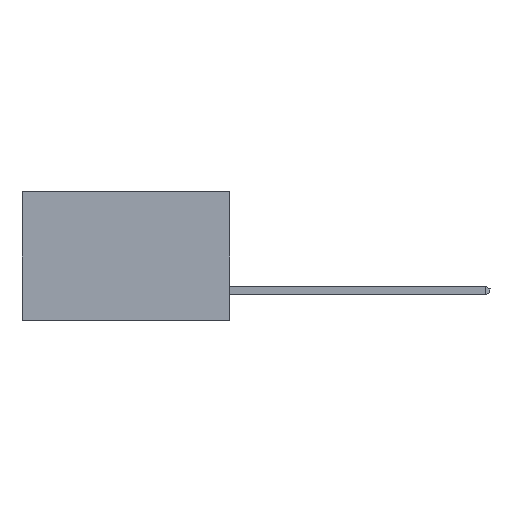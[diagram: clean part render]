
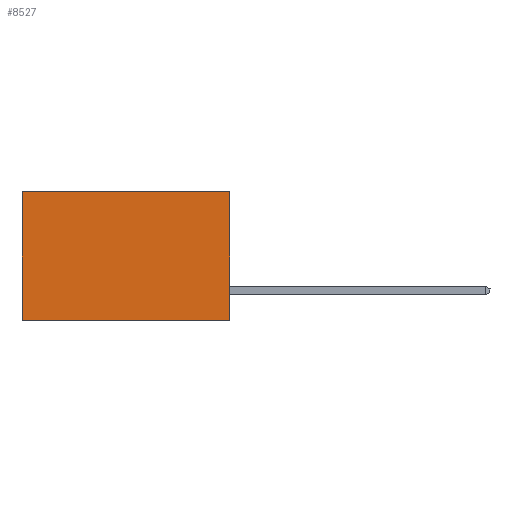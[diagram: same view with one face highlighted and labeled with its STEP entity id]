
A CAD part, left-side view. The second image highlights one B-rep face of the part: STEP entity #8527.
In plain terms, the highlighted planar face has unit normal (-1, 0, 0).
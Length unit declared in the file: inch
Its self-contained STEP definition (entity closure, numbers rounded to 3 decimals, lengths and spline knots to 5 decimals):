
#136 = LINE ( 'NONE', #9675, #4536 ) ;
#439 = VECTOR ( 'NONE', #9544, 39.37008 ) ;
#2019 = VERTEX_POINT ( 'NONE', #7161 ) ;
#2133 = FACE_OUTER_BOUND ( 'NONE', #12678, .T. ) ;
#2327 = ORIENTED_EDGE ( 'NONE', *, *, #19947, .F. ) ;
#3469 = VECTOR ( 'NONE', #21850, 39.37008 ) ;
#3531 = DIRECTION ( 'NONE',  ( 0., 1., 0. ) ) ;
#4450 = DIRECTION ( 'NONE',  ( 0., 0., -1. ) ) ;
#4536 = VECTOR ( 'NONE', #9619, 39.37008 ) ;
#5039 = DIRECTION ( 'NONE',  ( 1., 0., 0. ) ) ;
#5213 = CARTESIAN_POINT ( 'NONE',  ( 0.2615, 0.6, 0. ) ) ;
#5309 = CARTESIAN_POINT ( 'NONE',  ( 0.2615, 0., -0.37 ) ) ;
#5586 = CARTESIAN_POINT ( 'NONE',  ( 0.2615, 0., 0. ) ) ;
#6107 = PLANE ( 'NONE',  #15136 ) ;
#6421 = EDGE_CURVE ( 'NONE', #7771, #11549, #136, .T. ) ;
#7161 = CARTESIAN_POINT ( 'NONE',  ( 0.2615, 0., -0.37 ) ) ;
#7721 = CARTESIAN_POINT ( 'NONE',  ( 0.2615, 0., -0.37 ) ) ;
#7771 = VERTEX_POINT ( 'NONE', #5213 ) ;
#8527 = ADVANCED_FACE ( 'NONE', ( #2133 ), #6107, .F. ) ;
#9544 = DIRECTION ( 'NONE',  ( 0., 1., 0. ) ) ;
#9549 = ORIENTED_EDGE ( 'NONE', *, *, #15343, .T. ) ;
#9619 = DIRECTION ( 'NONE',  ( 0., 0., -1. ) ) ;
#9675 = CARTESIAN_POINT ( 'NONE',  ( 0.2615, 0.6, -0.37 ) ) ;
#10107 = VERTEX_POINT ( 'NONE', #5586 ) ;
#10223 = LINE ( 'NONE', #7721, #439 ) ;
#11531 = CARTESIAN_POINT ( 'NONE',  ( 0.2615, 0., -0.37 ) ) ;
#11549 = VERTEX_POINT ( 'NONE', #13173 ) ;
#12635 = ORIENTED_EDGE ( 'NONE', *, *, #13012, .F. ) ;
#12678 = EDGE_LOOP ( 'NONE', ( #15128, #2327, #12635, #9549 ) ) ;
#13012 = EDGE_CURVE ( 'NONE', #10107, #2019, #13165, .T. ) ;
#13165 = LINE ( 'NONE', #11531, #3469 ) ;
#13173 = CARTESIAN_POINT ( 'NONE',  ( 0.2615, 0.6, -0.37 ) ) ;
#14983 = LINE ( 'NONE', #16152, #20046 ) ;
#15128 = ORIENTED_EDGE ( 'NONE', *, *, #6421, .T. ) ;
#15136 = AXIS2_PLACEMENT_3D ( 'NONE', #5309, #5039, #4450 ) ;
#15343 = EDGE_CURVE ( 'NONE', #10107, #7771, #14983, .T. ) ;
#16152 = CARTESIAN_POINT ( 'NONE',  ( 0.2615, 0., 0. ) ) ;
#19947 = EDGE_CURVE ( 'NONE', #2019, #11549, #10223, .T. ) ;
#20046 = VECTOR ( 'NONE', #3531, 39.37008 ) ;
#21850 = DIRECTION ( 'NONE',  ( 0., 0., -1. ) ) ;
